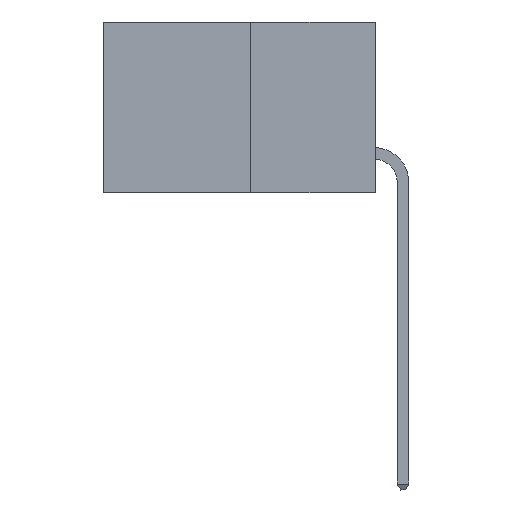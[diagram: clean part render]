
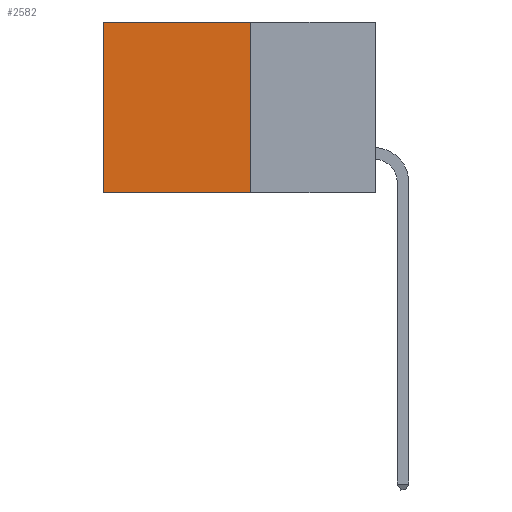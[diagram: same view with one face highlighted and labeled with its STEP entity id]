
A CAD part, left-side view. The second image highlights one B-rep face of the part: STEP entity #2582.
In plain terms, the highlighted planar face has unit normal (-1, 0, 0).
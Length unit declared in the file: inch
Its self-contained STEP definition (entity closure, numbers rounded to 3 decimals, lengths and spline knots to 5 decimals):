
#266 = FACE_OUTER_BOUND ( 'NONE', #1696, .T. ) ;
#381 = VECTOR ( 'NONE', #4607, 39.37008 ) ;
#717 = LINE ( 'NONE', #6770, #2741 ) ;
#1100 = EDGE_CURVE ( 'NONE', #4774, #8704, #5959, .T. ) ;
#1696 = EDGE_LOOP ( 'NONE', ( #2757, #2190, #1932, #8591 ) ) ;
#1932 = ORIENTED_EDGE ( 'NONE', *, *, #2161, .F. ) ;
#2093 = CARTESIAN_POINT ( 'NONE',  ( 0.277, 0.59, 0. ) ) ;
#2161 = EDGE_CURVE ( 'NONE', #4774, #7340, #4566, .T. ) ;
#2190 = ORIENTED_EDGE ( 'NONE', *, *, #3088, .F. ) ;
#2299 = CARTESIAN_POINT ( 'NONE',  ( 0.277, 0.27, 0. ) ) ;
#2466 = AXIS2_PLACEMENT_3D ( 'NONE', #4757, #4047, #4024 ) ;
#2582 = ADVANCED_FACE ( 'NONE', ( #266 ), #5470, .F. ) ;
#2741 = VECTOR ( 'NONE', #3791, 39.37008 ) ;
#2757 = ORIENTED_EDGE ( 'NONE', *, *, #7602, .T. ) ;
#3088 = EDGE_CURVE ( 'NONE', #7340, #6421, #3826, .T. ) ;
#3590 = CARTESIAN_POINT ( 'NONE',  ( 0.277, 0.27, -0.37 ) ) ;
#3791 = DIRECTION ( 'NONE',  ( 0., 0., -1. ) ) ;
#3826 = LINE ( 'NONE', #9258, #7803 ) ;
#4024 = DIRECTION ( 'NONE',  ( 0., 0., -1. ) ) ;
#4047 = DIRECTION ( 'NONE',  ( 1., 0., 0. ) ) ;
#4493 = CARTESIAN_POINT ( 'NONE',  ( 0.277, 0.27, 0. ) ) ;
#4566 = LINE ( 'NONE', #3590, #7832 ) ;
#4607 = DIRECTION ( 'NONE',  ( 0., 1., 0. ) ) ;
#4757 = CARTESIAN_POINT ( 'NONE',  ( 0.277, 0.27, -0.37 ) ) ;
#4763 = DIRECTION ( 'NONE',  ( 0., 1., 0. ) ) ;
#4774 = VERTEX_POINT ( 'NONE', #2299 ) ;
#5470 = PLANE ( 'NONE',  #2466 ) ;
#5959 = LINE ( 'NONE', #4493, #381 ) ;
#6421 = VERTEX_POINT ( 'NONE', #7567 ) ;
#6770 = CARTESIAN_POINT ( 'NONE',  ( 0.277, 0.59, -0.37 ) ) ;
#7270 = CARTESIAN_POINT ( 'NONE',  ( 0.277, 0.27, -0.37 ) ) ;
#7340 = VERTEX_POINT ( 'NONE', #7270 ) ;
#7567 = CARTESIAN_POINT ( 'NONE',  ( 0.277, 0.59, -0.37 ) ) ;
#7602 = EDGE_CURVE ( 'NONE', #8704, #6421, #717, .T. ) ;
#7803 = VECTOR ( 'NONE', #4763, 39.37008 ) ;
#7832 = VECTOR ( 'NONE', #8009, 39.37008 ) ;
#8009 = DIRECTION ( 'NONE',  ( 0., 0., -1. ) ) ;
#8591 = ORIENTED_EDGE ( 'NONE', *, *, #1100, .T. ) ;
#8704 = VERTEX_POINT ( 'NONE', #2093 ) ;
#9258 = CARTESIAN_POINT ( 'NONE',  ( 0.277, 0.27, -0.37 ) ) ;
